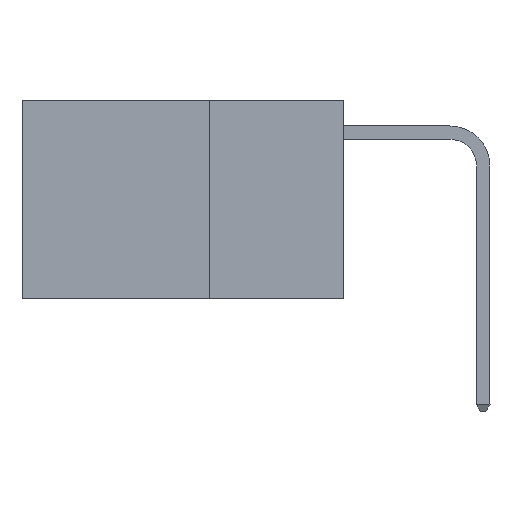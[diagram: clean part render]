
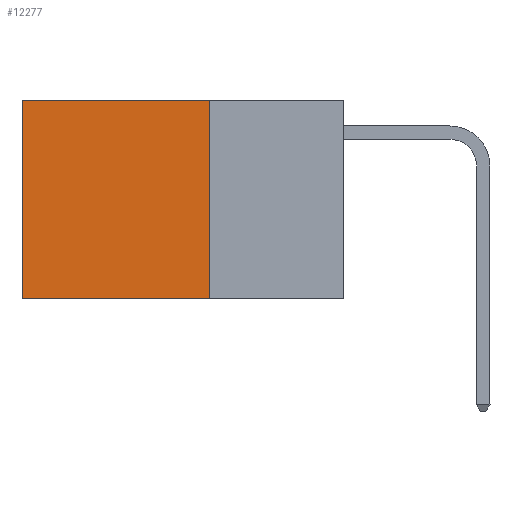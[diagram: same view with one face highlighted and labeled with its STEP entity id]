
A CAD part, left-side view. The second image highlights one B-rep face of the part: STEP entity #12277.
In plain terms, the highlighted planar face has unit normal (-1, 0, 0).
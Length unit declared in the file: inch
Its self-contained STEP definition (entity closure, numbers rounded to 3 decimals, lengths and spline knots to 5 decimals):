
#1102 = EDGE_CURVE ( 'NONE', #3106, #10037, #11843, .T. ) ;
#1317 = CARTESIAN_POINT ( 'NONE',  ( 0.2625, 0.25, 0. ) ) ;
#2112 = CARTESIAN_POINT ( 'NONE',  ( 0.2625, 0.25, 0. ) ) ;
#2711 = EDGE_LOOP ( 'NONE', ( #10273, #9456, #14051, #8618 ) ) ;
#3106 = VERTEX_POINT ( 'NONE', #13764 ) ;
#3120 = LINE ( 'NONE', #5822, #9252 ) ;
#3347 = DIRECTION ( 'NONE',  ( 0., 1., 0. ) ) ;
#4175 = CARTESIAN_POINT ( 'NONE',  ( 0.2625, 0.6, 0. ) ) ;
#4387 = VERTEX_POINT ( 'NONE', #4175 ) ;
#4422 = DIRECTION ( 'NONE',  ( 1., 0., 0. ) ) ;
#4461 = CARTESIAN_POINT ( 'NONE',  ( 0.2625, 0.25, 0. ) ) ;
#4700 = VECTOR ( 'NONE', #3347, 39.37008 ) ;
#4815 = AXIS2_PLACEMENT_3D ( 'NONE', #2112, #4422, #12285 ) ;
#4857 = CARTESIAN_POINT ( 'NONE',  ( 0.2625, 0.25, -0.37 ) ) ;
#4963 = FACE_OUTER_BOUND ( 'NONE', #2711, .T. ) ;
#5074 = LINE ( 'NONE', #4461, #4700 ) ;
#5553 = PLANE ( 'NONE',  #4815 ) ;
#5822 = CARTESIAN_POINT ( 'NONE',  ( 0.2625, 0.6, 0. ) ) ;
#6916 = VERTEX_POINT ( 'NONE', #13200 ) ;
#8095 = DIRECTION ( 'NONE',  ( 0., 0., -1. ) ) ;
#8406 = EDGE_CURVE ( 'NONE', #4387, #6916, #3120, .T. ) ;
#8435 = DIRECTION ( 'NONE',  ( 0., 0., -1. ) ) ;
#8470 = VECTOR ( 'NONE', #11625, 39.37008 ) ;
#8548 = VECTOR ( 'NONE', #8435, 39.37008 ) ;
#8618 = ORIENTED_EDGE ( 'NONE', *, *, #11298, .T. ) ;
#8835 = LINE ( 'NONE', #4857, #8470 ) ;
#9252 = VECTOR ( 'NONE', #8095, 39.37008 ) ;
#9456 = ORIENTED_EDGE ( 'NONE', *, *, #13881, .F. ) ;
#10037 = VERTEX_POINT ( 'NONE', #13547 ) ;
#10273 = ORIENTED_EDGE ( 'NONE', *, *, #8406, .T. ) ;
#11298 = EDGE_CURVE ( 'NONE', #3106, #4387, #5074, .T. ) ;
#11625 = DIRECTION ( 'NONE',  ( 0., 1., 0. ) ) ;
#11843 = LINE ( 'NONE', #1317, #8548 ) ;
#12277 = ADVANCED_FACE ( 'NONE', ( #4963 ), #5553, .F. ) ;
#12285 = DIRECTION ( 'NONE',  ( 0., 0., -1. ) ) ;
#13200 = CARTESIAN_POINT ( 'NONE',  ( 0.2625, 0.6, -0.37 ) ) ;
#13547 = CARTESIAN_POINT ( 'NONE',  ( 0.2625, 0.25, -0.37 ) ) ;
#13764 = CARTESIAN_POINT ( 'NONE',  ( 0.2625, 0.25, 0. ) ) ;
#13881 = EDGE_CURVE ( 'NONE', #10037, #6916, #8835, .T. ) ;
#14051 = ORIENTED_EDGE ( 'NONE', *, *, #1102, .F. ) ;
